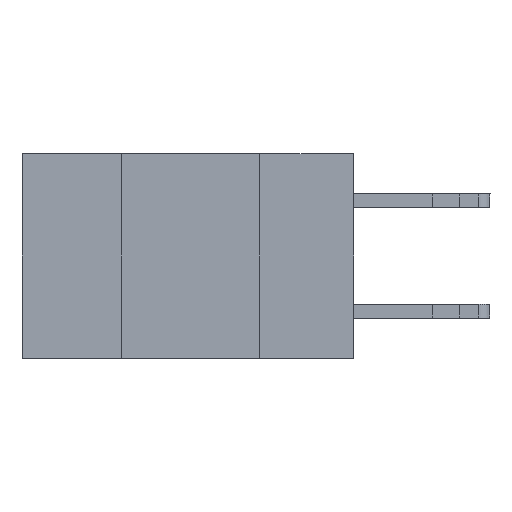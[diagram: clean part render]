
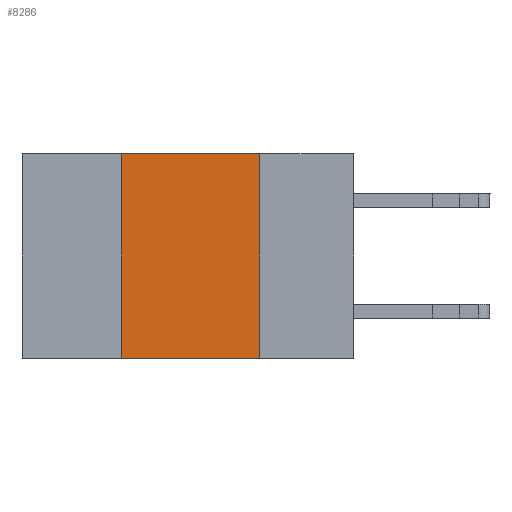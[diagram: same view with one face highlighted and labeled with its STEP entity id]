
A CAD part, left-side view. The second image highlights one B-rep face of the part: STEP entity #8286.
In plain terms, the highlighted planar face has unit normal (-1, 0, 0).
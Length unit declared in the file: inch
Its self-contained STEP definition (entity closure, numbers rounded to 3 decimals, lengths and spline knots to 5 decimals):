
#1386 = EDGE_LOOP ( 'NONE', ( #17919, #6837, #10387, #8540 ) ) ;
#1944 = VECTOR ( 'NONE', #6509, 39.37008 ) ;
#2047 = EDGE_CURVE ( 'NONE', #19828, #16410, #18810, .T. ) ;
#4337 = DIRECTION ( 'NONE',  ( 0., -1., 0. ) ) ;
#4392 = VERTEX_POINT ( 'NONE', #12840 ) ;
#4942 = DIRECTION ( 'NONE',  ( 0., 0., -1. ) ) ;
#6153 = CARTESIAN_POINT ( 'NONE',  ( 0., 0.17, 0. ) ) ;
#6156 = CARTESIAN_POINT ( 'NONE',  ( 0., 0.42, 0. ) ) ;
#6509 = DIRECTION ( 'NONE',  ( 0., -1., 0. ) ) ;
#6837 = ORIENTED_EDGE ( 'NONE', *, *, #18904, .F. ) ;
#7020 = VECTOR ( 'NONE', #15191, 39.37008 ) ;
#7138 = VERTEX_POINT ( 'NONE', #6153 ) ;
#7762 = CARTESIAN_POINT ( 'NONE',  ( 0., 0.6, -0.37 ) ) ;
#8286 = ADVANCED_FACE ( 'NONE', ( #14117 ), #17652, .F. ) ;
#8299 = CARTESIAN_POINT ( 'NONE',  ( 0., 0.42, -0.37 ) ) ;
#8540 = ORIENTED_EDGE ( 'NONE', *, *, #2047, .T. ) ;
#9787 = LINE ( 'NONE', #17642, #1944 ) ;
#10387 = ORIENTED_EDGE ( 'NONE', *, *, #15110, .F. ) ;
#10604 = CARTESIAN_POINT ( 'NONE',  ( 0., 0.17, -0.37 ) ) ;
#10865 = VECTOR ( 'NONE', #4337, 39.37008 ) ;
#12025 = EDGE_CURVE ( 'NONE', #7138, #16410, #20059, .T. ) ;
#12840 = CARTESIAN_POINT ( 'NONE',  ( 0., 0.42, 0. ) ) ;
#13431 = VECTOR ( 'NONE', #18544, 39.37008 ) ;
#13961 = AXIS2_PLACEMENT_3D ( 'NONE', #16294, #14330, #4942 ) ;
#14117 = FACE_OUTER_BOUND ( 'NONE', #1386, .T. ) ;
#14330 = DIRECTION ( 'NONE',  ( 1., 0., 0. ) ) ;
#15110 = EDGE_CURVE ( 'NONE', #19828, #4392, #18949, .T. ) ;
#15191 = DIRECTION ( 'NONE',  ( 0., 0., -1. ) ) ;
#16294 = CARTESIAN_POINT ( 'NONE',  ( 0., 0.6, 0. ) ) ;
#16410 = VERTEX_POINT ( 'NONE', #10604 ) ;
#16844 = CARTESIAN_POINT ( 'NONE',  ( 0., 0.17, 0. ) ) ;
#17642 = CARTESIAN_POINT ( 'NONE',  ( 0., 0.6, 0. ) ) ;
#17652 = PLANE ( 'NONE',  #13961 ) ;
#17919 = ORIENTED_EDGE ( 'NONE', *, *, #12025, .F. ) ;
#18544 = DIRECTION ( 'NONE',  ( 0., 0., 1. ) ) ;
#18810 = LINE ( 'NONE', #7762, #10865 ) ;
#18904 = EDGE_CURVE ( 'NONE', #4392, #7138, #9787, .T. ) ;
#18949 = LINE ( 'NONE', #6156, #13431 ) ;
#19828 = VERTEX_POINT ( 'NONE', #8299 ) ;
#20059 = LINE ( 'NONE', #16844, #7020 ) ;
